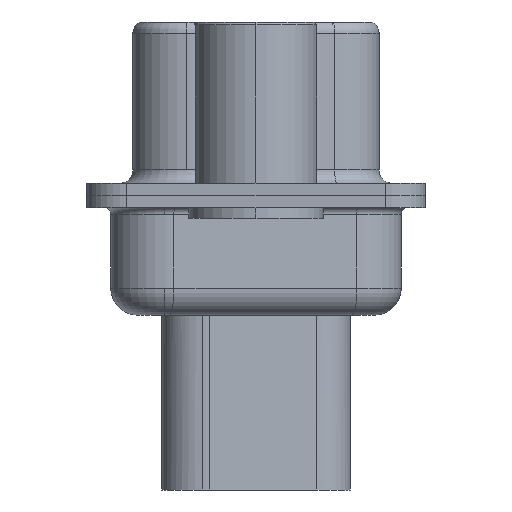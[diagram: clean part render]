
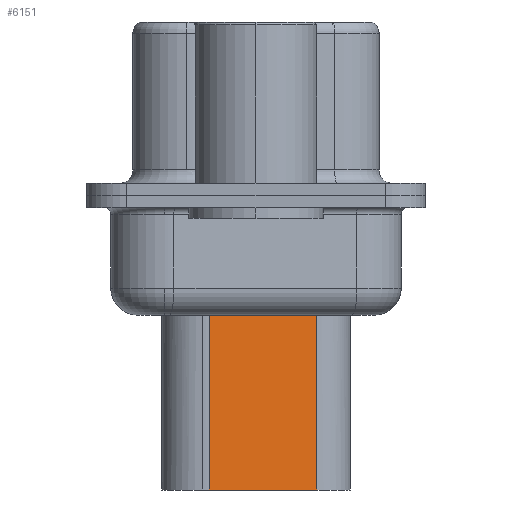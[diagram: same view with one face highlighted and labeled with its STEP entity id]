
A CAD part, left-side view. The second image highlights one B-rep face of the part: STEP entity #6151.
In plain terms, the highlighted planar face has unit normal (-0.985, -0.174, 0).
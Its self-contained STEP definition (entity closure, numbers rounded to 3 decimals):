
#3 = ORIENTED_EDGE ( 'NONE', *, *, #7273, .F. ) ;
#1242 = ORIENTED_EDGE ( 'NONE', *, *, #14357, .F. ) ;
#2906 = CARTESIAN_POINT ( 'NONE',  ( 4.524, 1.74, -3.1 ) ) ;
#3663 = VECTOR ( 'NONE', #10774, 1000. ) ;
#3866 = ORIENTED_EDGE ( 'NONE', *, *, #13768, .T. ) ;
#3942 = VERTEX_POINT ( 'NONE', #12159 ) ;
#4200 = DIRECTION ( 'NONE',  ( 0.174, -0.985, 0. ) ) ;
#4655 = FACE_OUTER_BOUND ( 'NONE', #17934, .T. ) ;
#5573 = CARTESIAN_POINT ( 'NONE',  ( 4.524, 1.74, -3.1 ) ) ;
#5674 = LINE ( 'NONE', #20148, #7571 ) ;
#5748 = VERTEX_POINT ( 'NONE', #17202 ) ;
#6151 = ADVANCED_FACE ( 'NONE', ( #4655 ), #16716, .T. ) ;
#7138 = VERTEX_POINT ( 'NONE', #9022 ) ;
#7273 = EDGE_CURVE ( 'NONE', #5748, #11280, #5674, .T. ) ;
#7571 = VECTOR ( 'NONE', #7738, 1000. ) ;
#7738 = DIRECTION ( 'NONE',  ( -0.174, 0.985, 0. ) ) ;
#7870 = DIRECTION ( 'NONE',  ( 0., 0., -1. ) ) ;
#8926 = LINE ( 'NONE', #10550, #13274 ) ;
#9022 = CARTESIAN_POINT ( 'NONE',  ( 4.524, 1.74, -3.975 ) ) ;
#9512 = DIRECTION ( 'NONE',  ( -0.985, -0.174, 0. ) ) ;
#10550 = CARTESIAN_POINT ( 'NONE',  ( 4.353, 2.709, -3.975 ) ) ;
#10774 = DIRECTION ( 'NONE',  ( 0., 0., -1. ) ) ;
#11280 = VERTEX_POINT ( 'NONE', #22405 ) ;
#11641 = AXIS2_PLACEMENT_3D ( 'NONE', #2906, #9512, #4200 ) ;
#12159 = CARTESIAN_POINT ( 'NONE',  ( 5.229, -2.26, -3.975 ) ) ;
#12912 = ORIENTED_EDGE ( 'NONE', *, *, #13627, .T. ) ;
#13274 = VECTOR ( 'NONE', #21095, 1000. ) ;
#13536 = LINE ( 'NONE', #16801, #21081 ) ;
#13627 = EDGE_CURVE ( 'NONE', #3942, #7138, #8926, .T. ) ;
#13768 = EDGE_CURVE ( 'NONE', #7138, #11280, #18203, .T. ) ;
#14357 = EDGE_CURVE ( 'NONE', #3942, #5748, #13536, .T. ) ;
#16716 = PLANE ( 'NONE',  #11641 ) ;
#16801 = CARTESIAN_POINT ( 'NONE',  ( 5.229, -2.26, -3.1 ) ) ;
#17202 = CARTESIAN_POINT ( 'NONE',  ( 5.229, -2.26, -10.95 ) ) ;
#17934 = EDGE_LOOP ( 'NONE', ( #1242, #12912, #3866, #3 ) ) ;
#18203 = LINE ( 'NONE', #5573, #3663 ) ;
#20148 = CARTESIAN_POINT ( 'NONE',  ( 4.524, 1.74, -10.95 ) ) ;
#21081 = VECTOR ( 'NONE', #7870, 1000. ) ;
#21095 = DIRECTION ( 'NONE',  ( -0.174, 0.985, 0. ) ) ;
#22405 = CARTESIAN_POINT ( 'NONE',  ( 4.524, 1.74, -10.95 ) ) ;
